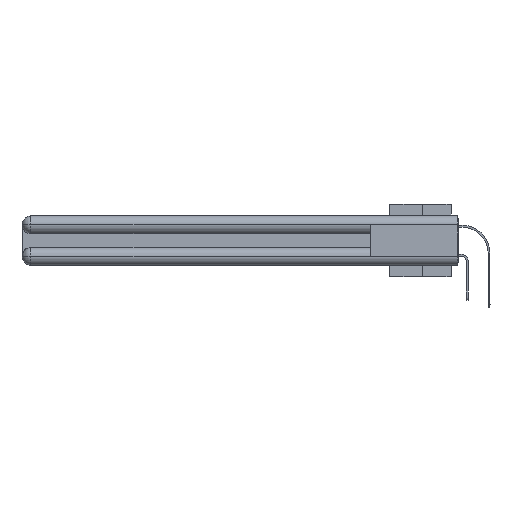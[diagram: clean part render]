
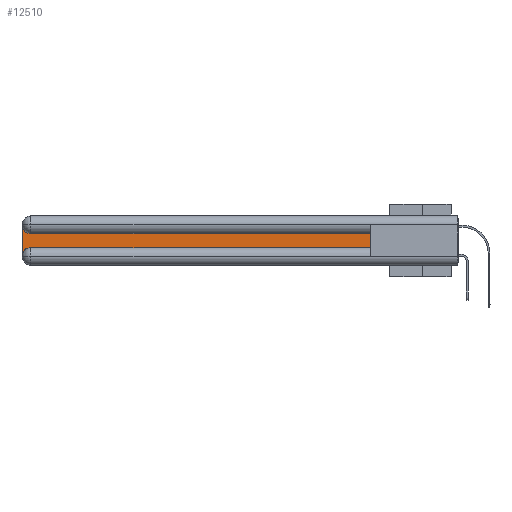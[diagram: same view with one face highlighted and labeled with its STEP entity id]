
A CAD part, left-side view. The second image highlights one B-rep face of the part: STEP entity #12510.
In plain terms, the highlighted planar face has unit normal (-1, 0, 0).
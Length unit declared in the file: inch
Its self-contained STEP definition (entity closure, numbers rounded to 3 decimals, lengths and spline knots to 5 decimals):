
#1335 = CARTESIAN_POINT ( 'NONE',  ( 0.075, 0.6, -0.2175 ) ) ;
#2564 = EDGE_LOOP ( 'NONE', ( #26088, #23817, #25836, #22336, #4534, #34393 ) ) ;
#4115 = VECTOR ( 'NONE', #24098, 39.37008 ) ;
#4534 = ORIENTED_EDGE ( 'NONE', *, *, #24687, .T. ) ;
#5310 = AXIS2_PLACEMENT_3D ( 'NONE', #28747, #14812, #25729 ) ;
#5342 = LINE ( 'NONE', #32159, #33812 ) ;
#5727 = DIRECTION ( 'NONE',  ( 1., 0., 0. ) ) ;
#5765 = EDGE_CURVE ( 'NONE', #18232, #28860, #5342, .T. ) ;
#5783 = EDGE_CURVE ( 'NONE', #16214, #18232, #13194, .T. ) ;
#5899 = VERTEX_POINT ( 'NONE', #22295 ) ;
#6882 = DIRECTION ( 'NONE',  ( 0., -1., 0. ) ) ;
#7537 = CARTESIAN_POINT ( 'NONE',  ( 0.075, 2.94, -0.0625 ) ) ;
#10233 = CARTESIAN_POINT ( 'NONE',  ( 0.075, 0.6, -0.1225 ) ) ;
#10734 = DIRECTION ( 'NONE',  ( 0., 0., -1. ) ) ;
#11006 = EDGE_CURVE ( 'NONE', #5899, #21709, #24120, .T. ) ;
#12510 = ADVANCED_FACE ( 'NONE', ( #34320 ), #23217, .F. ) ;
#13194 = LINE ( 'NONE', #34677, #4115 ) ;
#14812 = DIRECTION ( 'NONE',  ( 1., 0., 0. ) ) ;
#16143 = CARTESIAN_POINT ( 'NONE',  ( 0.075, 3., -0.2175 ) ) ;
#16214 = VERTEX_POINT ( 'NONE', #23141 ) ;
#16337 = DIRECTION ( 'NONE',  ( 0., 0., -1. ) ) ;
#16390 = EDGE_CURVE ( 'NONE', #26502, #5899, #21156, .T. ) ;
#18232 = VERTEX_POINT ( 'NONE', #10233 ) ;
#18749 = DIRECTION ( 'NONE',  ( 0., 1., 0. ) ) ;
#19122 = DIRECTION ( 'NONE',  ( 1., 0., 0. ) ) ;
#21156 = LINE ( 'NONE', #16143, #21999 ) ;
#21709 = VERTEX_POINT ( 'NONE', #32896 ) ;
#21999 = VECTOR ( 'NONE', #16337, 39.37008 ) ;
#22295 = CARTESIAN_POINT ( 'NONE',  ( 0.075, 3., -0.2775 ) ) ;
#22336 = ORIENTED_EDGE ( 'NONE', *, *, #11006, .T. ) ;
#23141 = CARTESIAN_POINT ( 'NONE',  ( 0.075, 0.6, -0.2175 ) ) ;
#23217 = PLANE ( 'NONE',  #5310 ) ;
#23376 = CIRCLE ( 'NONE', #27939, 0.06 ) ;
#23817 = ORIENTED_EDGE ( 'NONE', *, *, #25155, .T. ) ;
#24098 = DIRECTION ( 'NONE',  ( 0., 0., 1. ) ) ;
#24120 = CIRCLE ( 'NONE', #29847, 0.06 ) ;
#24687 = EDGE_CURVE ( 'NONE', #21709, #16214, #31901, .T. ) ;
#25155 = EDGE_CURVE ( 'NONE', #28860, #26502, #23376, .T. ) ;
#25179 = CARTESIAN_POINT ( 'NONE',  ( 0.075, 2.94, -0.2775 ) ) ;
#25729 = DIRECTION ( 'NONE',  ( 0., 0., -1. ) ) ;
#25836 = ORIENTED_EDGE ( 'NONE', *, *, #16390, .T. ) ;
#26088 = ORIENTED_EDGE ( 'NONE', *, *, #5765, .T. ) ;
#26502 = VERTEX_POINT ( 'NONE', #29334 ) ;
#27939 = AXIS2_PLACEMENT_3D ( 'NONE', #7537, #19122, #10734 ) ;
#28747 = CARTESIAN_POINT ( 'NONE',  ( 0.075, 3., -0.1225 ) ) ;
#28860 = VERTEX_POINT ( 'NONE', #29624 ) ;
#29071 = VECTOR ( 'NONE', #6882, 39.37008 ) ;
#29334 = CARTESIAN_POINT ( 'NONE',  ( 0.075, 3., -0.0625 ) ) ;
#29624 = CARTESIAN_POINT ( 'NONE',  ( 0.075, 2.94, -0.1225 ) ) ;
#29847 = AXIS2_PLACEMENT_3D ( 'NONE', #25179, #5727, #30370 ) ;
#30370 = DIRECTION ( 'NONE',  ( 0., 0., -1. ) ) ;
#31901 = LINE ( 'NONE', #1335, #29071 ) ;
#32159 = CARTESIAN_POINT ( 'NONE',  ( 0.075, 0.6, -0.1225 ) ) ;
#32896 = CARTESIAN_POINT ( 'NONE',  ( 0.075, 2.94, -0.2175 ) ) ;
#33812 = VECTOR ( 'NONE', #18749, 39.37008 ) ;
#34320 = FACE_OUTER_BOUND ( 'NONE', #2564, .T. ) ;
#34393 = ORIENTED_EDGE ( 'NONE', *, *, #5783, .T. ) ;
#34677 = CARTESIAN_POINT ( 'NONE',  ( 0.075, 0.6, -0.2175 ) ) ;
